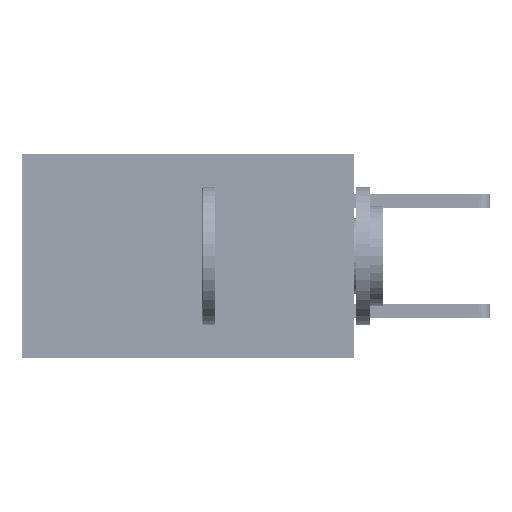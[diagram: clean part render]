
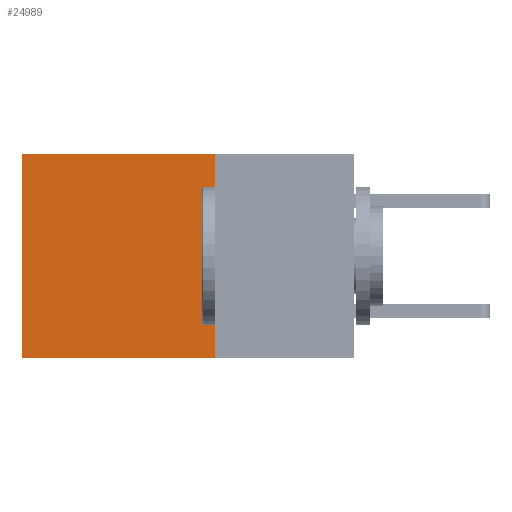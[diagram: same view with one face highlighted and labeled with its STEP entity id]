
A CAD part, left-side view. The second image highlights one B-rep face of the part: STEP entity #24989.
In plain terms, the highlighted planar face has unit normal (-1, 0, 0).
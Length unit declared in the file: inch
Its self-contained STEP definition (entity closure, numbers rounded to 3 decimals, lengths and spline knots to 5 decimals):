
#1242 = CARTESIAN_POINT ( 'NONE',  ( 0.2875, 0.25, -0.37 ) ) ;
#1607 = ORIENTED_EDGE ( 'NONE', *, *, #2572, .F. ) ;
#1610 = DIRECTION ( 'NONE',  ( 0., 0., -1. ) ) ;
#2572 = EDGE_CURVE ( 'NONE', #7928, #21115, #24990, .T. ) ;
#3788 = VECTOR ( 'NONE', #5818, 39.37008 ) ;
#4180 = AXIS2_PLACEMENT_3D ( 'NONE', #28293, #10401, #13437 ) ;
#4487 = CARTESIAN_POINT ( 'NONE',  ( 0.2875, 0.6, -0.37 ) ) ;
#5818 = DIRECTION ( 'NONE',  ( 0., 1., 0. ) ) ;
#6646 = CARTESIAN_POINT ( 'NONE',  ( 0.2875, 0.25, -0.37 ) ) ;
#7928 = VERTEX_POINT ( 'NONE', #6646 ) ;
#8872 = CARTESIAN_POINT ( 'NONE',  ( 0.2875, 0.25, 0. ) ) ;
#10401 = DIRECTION ( 'NONE',  ( 1., 0., 0. ) ) ;
#10581 = LINE ( 'NONE', #19978, #30034 ) ;
#11416 = LINE ( 'NONE', #8872, #3788 ) ;
#12212 = VERTEX_POINT ( 'NONE', #26999 ) ;
#12292 = LINE ( 'NONE', #23868, #31284 ) ;
#12650 = EDGE_CURVE ( 'NONE', #20204, #7928, #10581, .T. ) ;
#13437 = DIRECTION ( 'NONE',  ( 0., 0., -1. ) ) ;
#14975 = VECTOR ( 'NONE', #31262, 39.37008 ) ;
#17384 = ORIENTED_EDGE ( 'NONE', *, *, #27673, .T. ) ;
#18033 = CARTESIAN_POINT ( 'NONE',  ( 0.2875, 0.25, 0. ) ) ;
#19978 = CARTESIAN_POINT ( 'NONE',  ( 0.2875, 0.25, 0. ) ) ;
#20204 = VERTEX_POINT ( 'NONE', #18033 ) ;
#21115 = VERTEX_POINT ( 'NONE', #4487 ) ;
#21351 = DIRECTION ( 'NONE',  ( 0., 0., -1. ) ) ;
#23868 = CARTESIAN_POINT ( 'NONE',  ( 0.2875, 0.6, 0. ) ) ;
#24989 = ADVANCED_FACE ( 'NONE', ( #38229 ), #28557, .F. ) ;
#24990 = LINE ( 'NONE', #1242, #14975 ) ;
#26999 = CARTESIAN_POINT ( 'NONE',  ( 0.2875, 0.6, 0. ) ) ;
#27673 = EDGE_CURVE ( 'NONE', #20204, #12212, #11416, .T. ) ;
#28293 = CARTESIAN_POINT ( 'NONE',  ( 0.2875, 0.25, 0. ) ) ;
#28557 = PLANE ( 'NONE',  #4180 ) ;
#30034 = VECTOR ( 'NONE', #1610, 39.37008 ) ;
#31262 = DIRECTION ( 'NONE',  ( 0., 1., 0. ) ) ;
#31284 = VECTOR ( 'NONE', #21351, 39.37008 ) ;
#32876 = ORIENTED_EDGE ( 'NONE', *, *, #12650, .F. ) ;
#35906 = EDGE_LOOP ( 'NONE', ( #36726, #1607, #32876, #17384 ) ) ;
#36726 = ORIENTED_EDGE ( 'NONE', *, *, #38005, .T. ) ;
#38005 = EDGE_CURVE ( 'NONE', #12212, #21115, #12292, .T. ) ;
#38229 = FACE_OUTER_BOUND ( 'NONE', #35906, .T. ) ;
